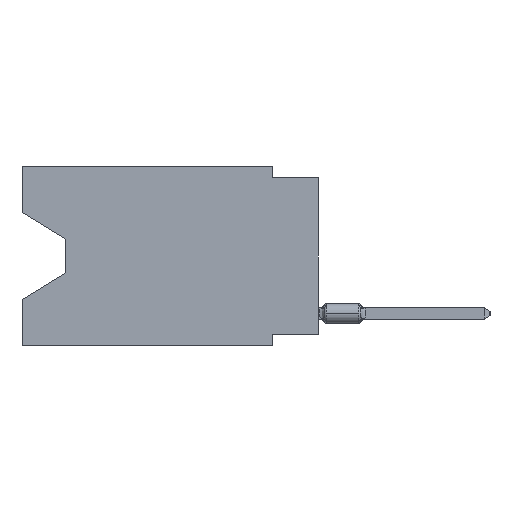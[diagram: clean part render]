
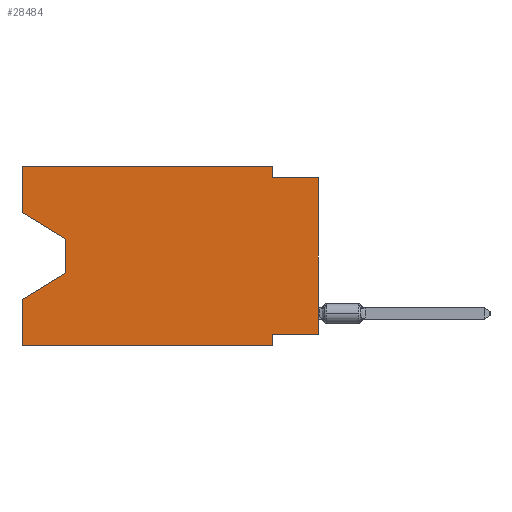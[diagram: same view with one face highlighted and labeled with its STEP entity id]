
A CAD part, left-side view. The second image highlights one B-rep face of the part: STEP entity #28484.
In plain terms, the highlighted planar face has unit normal (-1, 0, 0).
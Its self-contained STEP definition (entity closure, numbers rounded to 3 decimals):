
#242 = DIRECTION ( 'NONE',  ( 0., 0., 1. ) ) ;
#354 = DIRECTION ( 'NONE',  ( 1., 0., 0. ) ) ;
#1151 = CARTESIAN_POINT ( 'NONE',  ( 0., 2.54, -9.906 ) ) ;
#3128 = VERTEX_POINT ( 'NONE', #38450 ) ;
#3209 = EDGE_CURVE ( 'NONE', #19332, #52129, #44290, .T. ) ;
#3416 = EDGE_CURVE ( 'NONE', #31857, #19332, #7640, .T. ) ;
#3807 = DIRECTION ( 'NONE',  ( 0., -1., 0. ) ) ;
#4468 = VECTOR ( 'NONE', #41759, 1000. ) ;
#5391 = EDGE_CURVE ( 'NONE', #6810, #23205, #33449, .T. ) ;
#5575 = CARTESIAN_POINT ( 'NONE',  ( 0., 0., -9.271 ) ) ;
#5699 = DIRECTION ( 'NONE',  ( 0., 0., -1. ) ) ;
#6810 = VERTEX_POINT ( 'NONE', #12587 ) ;
#7640 = LINE ( 'NONE', #36744, #54201 ) ;
#7984 = AXIS2_PLACEMENT_3D ( 'NONE', #21618, #354, #47354 ) ;
#8343 = ORIENTED_EDGE ( 'NONE', *, *, #38933, .F. ) ;
#8567 = LINE ( 'NONE', #21146, #52239 ) ;
#9339 = ORIENTED_EDGE ( 'NONE', *, *, #3209, .F. ) ;
#11003 = ORIENTED_EDGE ( 'NONE', *, *, #21988, .T. ) ;
#11735 = CARTESIAN_POINT ( 'NONE',  ( 0., 13.97, -4.013 ) ) ;
#12074 = EDGE_CURVE ( 'NONE', #37660, #14665, #52562, .T. ) ;
#12331 = ORIENTED_EDGE ( 'NONE', *, *, #12546, .T. ) ;
#12546 = EDGE_CURVE ( 'NONE', #31857, #49130, #42750, .T. ) ;
#12587 = CARTESIAN_POINT ( 'NONE',  ( 0., 16.383, -2.546 ) ) ;
#13336 = VECTOR ( 'NONE', #51781, 1000. ) ;
#14440 = DIRECTION ( 'NONE',  ( 0., 0., -1. ) ) ;
#14481 = EDGE_CURVE ( 'NONE', #29098, #14665, #48944, .T. ) ;
#14665 = VERTEX_POINT ( 'NONE', #42460 ) ;
#15453 = VECTOR ( 'NONE', #18765, 1000. ) ;
#16183 = VECTOR ( 'NONE', #50353, 1000. ) ;
#17717 = CARTESIAN_POINT ( 'NONE',  ( 0., 16.383, 0. ) ) ;
#18765 = DIRECTION ( 'NONE',  ( 0., 0.855, -0.519 ) ) ;
#19332 = VERTEX_POINT ( 'NONE', #53238 ) ;
#19651 = ORIENTED_EDGE ( 'NONE', *, *, #14481, .F. ) ;
#20029 = CARTESIAN_POINT ( 'NONE',  ( 0., 2.54, 0. ) ) ;
#20234 = CARTESIAN_POINT ( 'NONE',  ( 0., 0., -0.635 ) ) ;
#21146 = CARTESIAN_POINT ( 'NONE',  ( 0., 16.383, -9.906 ) ) ;
#21479 = CARTESIAN_POINT ( 'NONE',  ( 0., 0., -0.635 ) ) ;
#21618 = CARTESIAN_POINT ( 'NONE',  ( 0., 16.383, 0. ) ) ;
#21988 = EDGE_CURVE ( 'NONE', #29098, #52129, #8567, .T. ) ;
#22174 = LINE ( 'NONE', #17717, #13336 ) ;
#22234 = VECTOR ( 'NONE', #26003, 1000. ) ;
#23205 = VERTEX_POINT ( 'NONE', #11735 ) ;
#23785 = DIRECTION ( 'NONE',  ( 0., 0., 1. ) ) ;
#24712 = DIRECTION ( 'NONE',  ( 0., 1., 0. ) ) ;
#26003 = DIRECTION ( 'NONE',  ( 0., 0., 1. ) ) ;
#26566 = VECTOR ( 'NONE', #5699, 1000. ) ;
#28400 = CARTESIAN_POINT ( 'NONE',  ( 0., 16.383, -2.546 ) ) ;
#28474 = EDGE_CURVE ( 'NONE', #3128, #39955, #22174, .T. ) ;
#28484 = ADVANCED_FACE ( 'NONE', ( #34217 ), #51243, .F. ) ;
#29098 = VERTEX_POINT ( 'NONE', #54469 ) ;
#30800 = ORIENTED_EDGE ( 'NONE', *, *, #48473, .T. ) ;
#31445 = ORIENTED_EDGE ( 'NONE', *, *, #28474, .F. ) ;
#31716 = EDGE_CURVE ( 'NONE', #6810, #3128, #42240, .T. ) ;
#31857 = VERTEX_POINT ( 'NONE', #5575 ) ;
#31935 = LINE ( 'NONE', #48985, #16183 ) ;
#32444 = CARTESIAN_POINT ( 'NONE',  ( 0., 16.383, 0. ) ) ;
#32479 = CARTESIAN_POINT ( 'NONE',  ( 0., 2.54, -0.635 ) ) ;
#33449 = LINE ( 'NONE', #28400, #33778 ) ;
#33778 = VECTOR ( 'NONE', #54098, 1000. ) ;
#34217 = FACE_OUTER_BOUND ( 'NONE', #37557, .T. ) ;
#35268 = VECTOR ( 'NONE', #23785, 1000. ) ;
#35342 = CARTESIAN_POINT ( 'NONE',  ( 0., 2.54, -9.906 ) ) ;
#35813 = CARTESIAN_POINT ( 'NONE',  ( 0., 13.97, -5.893 ) ) ;
#36254 = LINE ( 'NONE', #20029, #44296 ) ;
#36744 = CARTESIAN_POINT ( 'NONE',  ( 0., 0., -9.271 ) ) ;
#37557 = EDGE_LOOP ( 'NONE', ( #45058, #30800, #53300, #19651, #11003, #9339, #45464, #12331, #8343, #42255, #31445, #49893 ) ) ;
#37571 = LINE ( 'NONE', #20234, #4468 ) ;
#37660 = VERTEX_POINT ( 'NONE', #53201 ) ;
#38450 = CARTESIAN_POINT ( 'NONE',  ( 0., 16.383, 0. ) ) ;
#38933 = EDGE_CURVE ( 'NONE', #53404, #49130, #37571, .T. ) ;
#39955 = VERTEX_POINT ( 'NONE', #53133 ) ;
#41759 = DIRECTION ( 'NONE',  ( 0., -1., 0. ) ) ;
#42046 = EDGE_CURVE ( 'NONE', #39955, #53404, #36254, .T. ) ;
#42240 = LINE ( 'NONE', #46717, #22234 ) ;
#42255 = ORIENTED_EDGE ( 'NONE', *, *, #42046, .F. ) ;
#42460 = CARTESIAN_POINT ( 'NONE',  ( 0., 16.383, -7.36 ) ) ;
#42750 = LINE ( 'NONE', #53246, #53810 ) ;
#44290 = LINE ( 'NONE', #35342, #26566 ) ;
#44296 = VECTOR ( 'NONE', #14440, 1000. ) ;
#45058 = ORIENTED_EDGE ( 'NONE', *, *, #5391, .T. ) ;
#45464 = ORIENTED_EDGE ( 'NONE', *, *, #3416, .F. ) ;
#46717 = CARTESIAN_POINT ( 'NONE',  ( 0., 16.383, 0. ) ) ;
#47354 = DIRECTION ( 'NONE',  ( 0., 0., -1. ) ) ;
#48473 = EDGE_CURVE ( 'NONE', #23205, #37660, #31935, .T. ) ;
#48944 = LINE ( 'NONE', #32444, #35268 ) ;
#48985 = CARTESIAN_POINT ( 'NONE',  ( 0., 13.97, -4.013 ) ) ;
#49130 = VERTEX_POINT ( 'NONE', #21479 ) ;
#49893 = ORIENTED_EDGE ( 'NONE', *, *, #31716, .F. ) ;
#50353 = DIRECTION ( 'NONE',  ( 0., 0., -1. ) ) ;
#51243 = PLANE ( 'NONE',  #7984 ) ;
#51781 = DIRECTION ( 'NONE',  ( 0., -1., 0. ) ) ;
#52129 = VERTEX_POINT ( 'NONE', #1151 ) ;
#52239 = VECTOR ( 'NONE', #3807, 1000. ) ;
#52562 = LINE ( 'NONE', #35813, #15453 ) ;
#53133 = CARTESIAN_POINT ( 'NONE',  ( 0., 2.54, 0. ) ) ;
#53201 = CARTESIAN_POINT ( 'NONE',  ( 0., 13.97, -5.893 ) ) ;
#53238 = CARTESIAN_POINT ( 'NONE',  ( 0., 2.54, -9.271 ) ) ;
#53246 = CARTESIAN_POINT ( 'NONE',  ( 0., 0., 0. ) ) ;
#53300 = ORIENTED_EDGE ( 'NONE', *, *, #12074, .T. ) ;
#53404 = VERTEX_POINT ( 'NONE', #32479 ) ;
#53810 = VECTOR ( 'NONE', #242, 1000. ) ;
#54098 = DIRECTION ( 'NONE',  ( 0., -0.855, -0.519 ) ) ;
#54201 = VECTOR ( 'NONE', #24712, 1000. ) ;
#54469 = CARTESIAN_POINT ( 'NONE',  ( 0., 16.383, -9.906 ) ) ;
